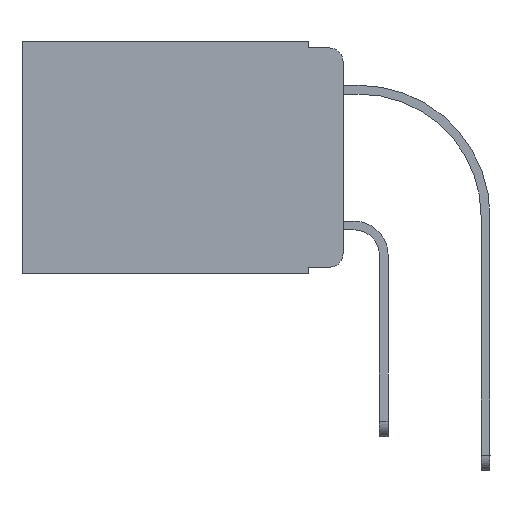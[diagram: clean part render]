
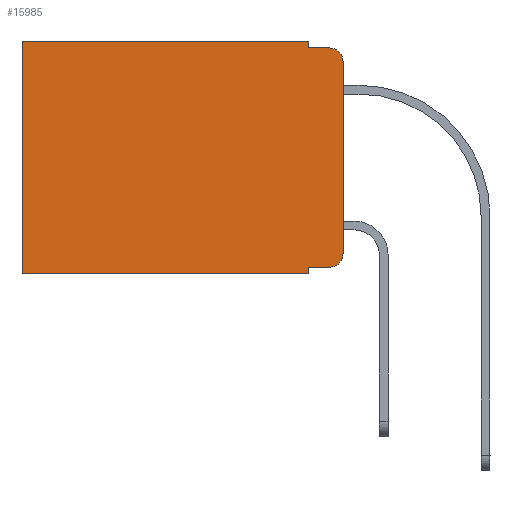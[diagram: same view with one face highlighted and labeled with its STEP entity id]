
A CAD part, left-side view. The second image highlights one B-rep face of the part: STEP entity #15985.
In plain terms, the highlighted planar face has unit normal (-1, 0, 0).
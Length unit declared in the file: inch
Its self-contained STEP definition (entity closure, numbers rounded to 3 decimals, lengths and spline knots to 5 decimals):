
#418 = VERTEX_POINT ( 'NONE', #12913 ) ;
#448 = VERTEX_POINT ( 'NONE', #3990 ) ;
#1042 = CARTESIAN_POINT ( 'NONE',  ( 0.298, 0., 0. ) ) ;
#1626 = VECTOR ( 'NONE', #5609, 39.37008 ) ;
#2277 = LINE ( 'NONE', #16499, #21105 ) ;
#2352 = EDGE_CURVE ( 'NONE', #448, #6571, #15269, .T. ) ;
#2572 = VERTEX_POINT ( 'NONE', #3832 ) ;
#2869 = VECTOR ( 'NONE', #21003, 39.37008 ) ;
#2891 = FACE_OUTER_BOUND ( 'NONE', #8083, .T. ) ;
#3413 = VERTEX_POINT ( 'NONE', #19074 ) ;
#3492 = VECTOR ( 'NONE', #14586, 39.37008 ) ;
#3821 = DIRECTION ( 'NONE',  ( 0., -1., 0. ) ) ;
#3832 = CARTESIAN_POINT ( 'NONE',  ( 0.298, 0.051, -0.01 ) ) ;
#3990 = CARTESIAN_POINT ( 'NONE',  ( 0.298, 0., -0.03 ) ) ;
#4053 = VERTEX_POINT ( 'NONE', #16775 ) ;
#4554 = DIRECTION ( 'NONE',  ( 0., 1., 0. ) ) ;
#5332 = CIRCLE ( 'NONE', #19594, 0.02 ) ;
#5609 = DIRECTION ( 'NONE',  ( 0., 1., 0. ) ) ;
#5737 = AXIS2_PLACEMENT_3D ( 'NONE', #13247, #22423, #9970 ) ;
#6084 = LINE ( 'NONE', #1042, #18188 ) ;
#6571 = VERTEX_POINT ( 'NONE', #14494 ) ;
#6574 = CARTESIAN_POINT ( 'NONE',  ( 0.298, 0.051, -0.333 ) ) ;
#6886 = AXIS2_PLACEMENT_3D ( 'NONE', #10054, #12151, #19325 ) ;
#7381 = LINE ( 'NONE', #21711, #1626 ) ;
#7413 = CARTESIAN_POINT ( 'NONE',  ( 0.298, 0.051, 0. ) ) ;
#7929 = ORIENTED_EDGE ( 'NONE', *, *, #11963, .T. ) ;
#8057 = CARTESIAN_POINT ( 'NONE',  ( 0.298, 0.02, -0.03 ) ) ;
#8083 = EDGE_LOOP ( 'NONE', ( #20329, #16290, #20349, #11094, #22551, #11010, #19349, #20793, #10978, #7929 ) ) ;
#8177 = CARTESIAN_POINT ( 'NONE',  ( 0.298, 0.473, 0. ) ) ;
#8396 = LINE ( 'NONE', #8177, #10632 ) ;
#9111 = LINE ( 'NONE', #19810, #15507 ) ;
#9970 = DIRECTION ( 'NONE',  ( 0., 0., -1. ) ) ;
#10054 = CARTESIAN_POINT ( 'NONE',  ( 0.298, 0., 0. ) ) ;
#10278 = DIRECTION ( 'NONE',  ( 0., 0., -1. ) ) ;
#10545 = EDGE_CURVE ( 'NONE', #20552, #19859, #7381, .T. ) ;
#10632 = VECTOR ( 'NONE', #10278, 39.37008 ) ;
#10978 = ORIENTED_EDGE ( 'NONE', *, *, #13134, .T. ) ;
#11010 = ORIENTED_EDGE ( 'NONE', *, *, #15895, .T. ) ;
#11094 = ORIENTED_EDGE ( 'NONE', *, *, #15347, .F. ) ;
#11380 = CARTESIAN_POINT ( 'NONE',  ( 0.298, 0.473, -0.343 ) ) ;
#11732 = DIRECTION ( 'NONE',  ( 0., -1., 0. ) ) ;
#11963 = EDGE_CURVE ( 'NONE', #418, #6571, #18111, .T. ) ;
#12151 = DIRECTION ( 'NONE',  ( 1., 0., 0. ) ) ;
#12913 = CARTESIAN_POINT ( 'NONE',  ( 0.298, 0.02, -0.333 ) ) ;
#13134 = EDGE_CURVE ( 'NONE', #20679, #418, #22671, .T. ) ;
#13247 = CARTESIAN_POINT ( 'NONE',  ( 0.298, 0.02, -0.313 ) ) ;
#13460 = DIRECTION ( 'NONE',  ( -1., 0., 0. ) ) ;
#13614 = CARTESIAN_POINT ( 'NONE',  ( 0.298, 0., 0. ) ) ;
#13808 = PLANE ( 'NONE',  #6886 ) ;
#14494 = CARTESIAN_POINT ( 'NONE',  ( 0.298, 0., -0.313 ) ) ;
#14570 = EDGE_CURVE ( 'NONE', #448, #18402, #5332, .T. ) ;
#14586 = DIRECTION ( 'NONE',  ( 0., 0., -1. ) ) ;
#14902 = EDGE_CURVE ( 'NONE', #20679, #20552, #2277, .T. ) ;
#15269 = LINE ( 'NONE', #13614, #2869 ) ;
#15347 = EDGE_CURVE ( 'NONE', #3413, #2572, #16472, .T. ) ;
#15507 = VECTOR ( 'NONE', #3821, 39.37008 ) ;
#15676 = EDGE_CURVE ( 'NONE', #2572, #18402, #9111, .T. ) ;
#15895 = EDGE_CURVE ( 'NONE', #4053, #19859, #8396, .T. ) ;
#15934 = VECTOR ( 'NONE', #11732, 39.37008 ) ;
#15985 = ADVANCED_FACE ( 'NONE', ( #2891 ), #13808, .F. ) ;
#16079 = CARTESIAN_POINT ( 'NONE',  ( 0.298, 0.02, -0.01 ) ) ;
#16290 = ORIENTED_EDGE ( 'NONE', *, *, #14570, .T. ) ;
#16472 = LINE ( 'NONE', #7413, #3492 ) ;
#16499 = CARTESIAN_POINT ( 'NONE',  ( 0.298, 0.051, 0. ) ) ;
#16775 = CARTESIAN_POINT ( 'NONE',  ( 0.298, 0.473, 0. ) ) ;
#16941 = CARTESIAN_POINT ( 'NONE',  ( 0.298, 0.051, -0.333 ) ) ;
#17152 = EDGE_CURVE ( 'NONE', #3413, #4053, #6084, .T. ) ;
#18111 = CIRCLE ( 'NONE', #5737, 0.02 ) ;
#18188 = VECTOR ( 'NONE', #4554, 39.37008 ) ;
#18402 = VERTEX_POINT ( 'NONE', #16079 ) ;
#19074 = CARTESIAN_POINT ( 'NONE',  ( 0.298, 0.051, 0. ) ) ;
#19325 = DIRECTION ( 'NONE',  ( 0., 0., -1. ) ) ;
#19349 = ORIENTED_EDGE ( 'NONE', *, *, #10545, .F. ) ;
#19594 = AXIS2_PLACEMENT_3D ( 'NONE', #8057, #13460, #20621 ) ;
#19649 = CARTESIAN_POINT ( 'NONE',  ( 0.298, 0.051, -0.343 ) ) ;
#19810 = CARTESIAN_POINT ( 'NONE',  ( 0.298, 0.051, -0.01 ) ) ;
#19859 = VERTEX_POINT ( 'NONE', #11380 ) ;
#20329 = ORIENTED_EDGE ( 'NONE', *, *, #2352, .F. ) ;
#20349 = ORIENTED_EDGE ( 'NONE', *, *, #15676, .F. ) ;
#20552 = VERTEX_POINT ( 'NONE', #19649 ) ;
#20621 = DIRECTION ( 'NONE',  ( 0., 0., -1. ) ) ;
#20679 = VERTEX_POINT ( 'NONE', #16941 ) ;
#20793 = ORIENTED_EDGE ( 'NONE', *, *, #14902, .F. ) ;
#21003 = DIRECTION ( 'NONE',  ( 0., 0., -1. ) ) ;
#21105 = VECTOR ( 'NONE', #21885, 39.37008 ) ;
#21711 = CARTESIAN_POINT ( 'NONE',  ( 0.298, 0., -0.343 ) ) ;
#21885 = DIRECTION ( 'NONE',  ( 0., 0., -1. ) ) ;
#22423 = DIRECTION ( 'NONE',  ( -1., 0., 0. ) ) ;
#22551 = ORIENTED_EDGE ( 'NONE', *, *, #17152, .T. ) ;
#22671 = LINE ( 'NONE', #6574, #15934 ) ;
